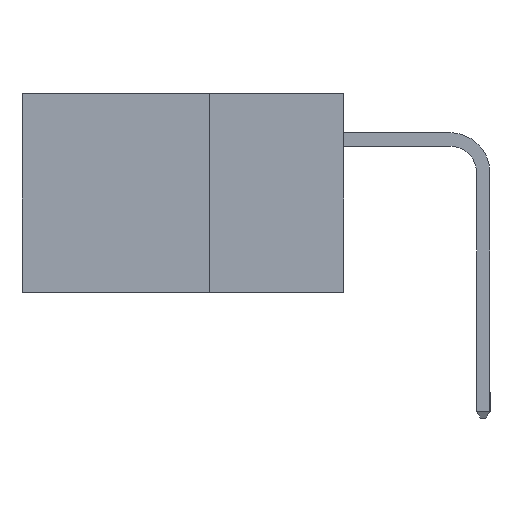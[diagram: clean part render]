
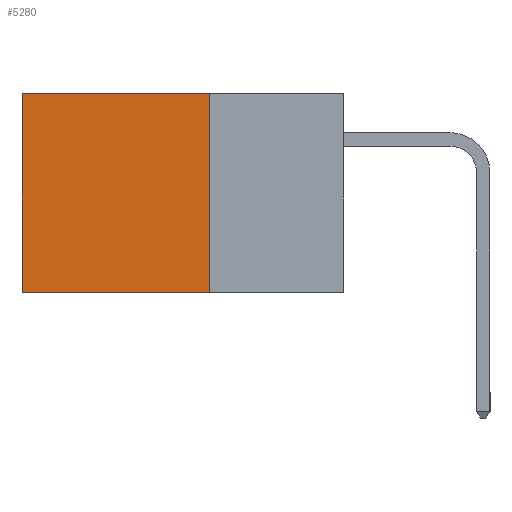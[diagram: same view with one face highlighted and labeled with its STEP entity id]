
A CAD part, left-side view. The second image highlights one B-rep face of the part: STEP entity #5280.
In plain terms, the highlighted planar face has unit normal (-1, 0, 0).
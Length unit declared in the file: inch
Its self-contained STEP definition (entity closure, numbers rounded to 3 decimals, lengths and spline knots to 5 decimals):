
#391 = CARTESIAN_POINT ( 'NONE',  ( 0.298, 0.25, -0.37 ) ) ;
#449 = LINE ( 'NONE', #11644, #9734 ) ;
#656 = EDGE_LOOP ( 'NONE', ( #8607, #9703, #4976, #824 ) ) ;
#824 = ORIENTED_EDGE ( 'NONE', *, *, #9055, .T. ) ;
#1884 = VECTOR ( 'NONE', #9318, 39.37008 ) ;
#2361 = VERTEX_POINT ( 'NONE', #9983 ) ;
#2408 = CARTESIAN_POINT ( 'NONE',  ( 0.298, 0.25, 0. ) ) ;
#3439 = VERTEX_POINT ( 'NONE', #9425 ) ;
#4231 = EDGE_CURVE ( 'NONE', #5129, #2361, #449, .T. ) ;
#4637 = DIRECTION ( 'NONE',  ( 0., 0., -1. ) ) ;
#4671 = DIRECTION ( 'NONE',  ( 1., 0., 0. ) ) ;
#4692 = CARTESIAN_POINT ( 'NONE',  ( 0.298, 0.25, 0. ) ) ;
#4852 = PLANE ( 'NONE',  #6076 ) ;
#4976 = ORIENTED_EDGE ( 'NONE', *, *, #9444, .F. ) ;
#5129 = VERTEX_POINT ( 'NONE', #7030 ) ;
#5138 = VECTOR ( 'NONE', #7401, 39.37008 ) ;
#5280 = ADVANCED_FACE ( 'NONE', ( #13992 ), #4852, .F. ) ;
#5552 = LINE ( 'NONE', #12191, #1884 ) ;
#5592 = EDGE_CURVE ( 'NONE', #3439, #2361, #12920, .T. ) ;
#5765 = DIRECTION ( 'NONE',  ( 0., 1., 0. ) ) ;
#5992 = LINE ( 'NONE', #11292, #16538 ) ;
#6076 = AXIS2_PLACEMENT_3D ( 'NONE', #4692, #4671, #4637 ) ;
#6886 = VERTEX_POINT ( 'NONE', #2408 ) ;
#7030 = CARTESIAN_POINT ( 'NONE',  ( 0.298, 0.6, 0. ) ) ;
#7401 = DIRECTION ( 'NONE',  ( 0., 1., 0. ) ) ;
#8607 = ORIENTED_EDGE ( 'NONE', *, *, #4231, .T. ) ;
#9055 = EDGE_CURVE ( 'NONE', #6886, #5129, #5992, .T. ) ;
#9318 = DIRECTION ( 'NONE',  ( 0., 0., -1. ) ) ;
#9425 = CARTESIAN_POINT ( 'NONE',  ( 0.298, 0.25, -0.37 ) ) ;
#9444 = EDGE_CURVE ( 'NONE', #6886, #3439, #5552, .T. ) ;
#9703 = ORIENTED_EDGE ( 'NONE', *, *, #5592, .F. ) ;
#9734 = VECTOR ( 'NONE', #12086, 39.37008 ) ;
#9983 = CARTESIAN_POINT ( 'NONE',  ( 0.298, 0.6, -0.37 ) ) ;
#11292 = CARTESIAN_POINT ( 'NONE',  ( 0.298, 0.25, 0. ) ) ;
#11644 = CARTESIAN_POINT ( 'NONE',  ( 0.298, 0.6, 0. ) ) ;
#12086 = DIRECTION ( 'NONE',  ( 0., 0., -1. ) ) ;
#12191 = CARTESIAN_POINT ( 'NONE',  ( 0.298, 0.25, 0. ) ) ;
#12920 = LINE ( 'NONE', #391, #5138 ) ;
#13992 = FACE_OUTER_BOUND ( 'NONE', #656, .T. ) ;
#16538 = VECTOR ( 'NONE', #5765, 39.37008 ) ;
